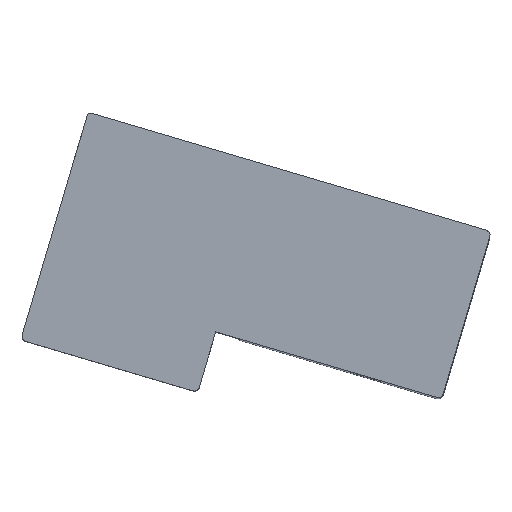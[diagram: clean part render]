
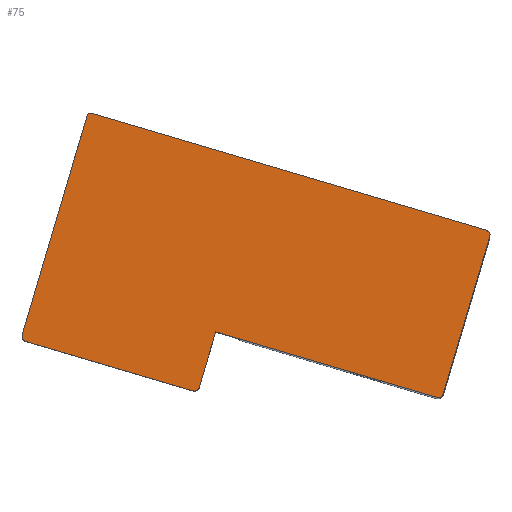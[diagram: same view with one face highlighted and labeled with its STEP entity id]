
A CAD part, top view. The second image highlights one B-rep face of the part: STEP entity #75.
In plain terms, the highlighted planar face has unit normal (0, 0, 1).
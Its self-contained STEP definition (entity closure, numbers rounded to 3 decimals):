
#22 = DIRECTION ( 'NONE',  ( 0., 0., -1. ) ) ;
#32 = EDGE_CURVE ( 'NONE', #1197, #1058, #312, .T. ) ;
#64 = ORIENTED_EDGE ( 'NONE', *, *, #1459, .F. ) ;
#72 = DIRECTION ( 'NONE',  ( -0.477, 0.879, 0. ) ) ;
#73 = DIRECTION ( 'NONE',  ( 0., 0., -1. ) ) ;
#75 = ADVANCED_FACE ( 'NONE', ( #539 ), #894, .F. ) ;
#135 = VECTOR ( 'NONE', #1700, 1000. ) ;
#195 = AXIS2_PLACEMENT_3D ( 'NONE', #910, #1368, #1363 ) ;
#199 = AXIS2_PLACEMENT_3D ( 'NONE', #1148, #73, #1041 ) ;
#220 = CIRCLE ( 'NONE', #1052, 0.15 ) ;
#256 = CARTESIAN_POINT ( 'NONE',  ( -35.314, -26.696, 19. ) ) ;
#312 = LINE ( 'NONE', #2003, #135 ) ;
#317 = EDGE_CURVE ( 'NONE', #1906, #722, #1544, .T. ) ;
#335 = VERTEX_POINT ( 'NONE', #377 ) ;
#338 = VERTEX_POINT ( 'NONE', #691 ) ;
#373 = VECTOR ( 'NONE', #1524, 1000. ) ;
#377 = CARTESIAN_POINT ( 'NONE',  ( -45.306, -26.891, 19. ) ) ;
#398 = VECTOR ( 'NONE', #870, 1000. ) ;
#465 = EDGE_CURVE ( 'NONE', #752, #1354, #775, .T. ) ;
#474 = CARTESIAN_POINT ( 'NONE',  ( -25.535, -29.332, 19. ) ) ;
#512 = AXIS2_PLACEMENT_3D ( 'NONE', #1888, #1242, #793 ) ;
#537 = ORIENTED_EDGE ( 'NONE', *, *, #1115, .F. ) ;
#539 = FACE_OUTER_BOUND ( 'NONE', #1815, .T. ) ;
#614 = CARTESIAN_POINT ( 'NONE',  ( -25.295, -29.403, 19. ) ) ;
#615 = ORIENTED_EDGE ( 'NONE', *, *, #727, .F. ) ;
#625 = LINE ( 'NONE', #635, #853 ) ;
#635 = CARTESIAN_POINT ( 'NONE',  ( -32.945, -18.688, 19. ) ) ;
#640 = DIRECTION ( 'NONE',  ( 0., 0., -1. ) ) ;
#643 = CARTESIAN_POINT ( 'NONE',  ( -25.606, -29.571, 19. ) ) ;
#646 = DIRECTION ( 'NONE',  ( 0.477, -0.879, 0. ) ) ;
#691 = CARTESIAN_POINT ( 'NONE',  ( -23.234, -21.565, 19. ) ) ;
#705 = CARTESIAN_POINT ( 'NONE',  ( -37.3, -29.262, 19. ) ) ;
#707 = VECTOR ( 'NONE', #1489, 1000. ) ;
#713 = CARTESIAN_POINT ( 'NONE',  ( -41.174, -12.062, 19. ) ) ;
#722 = VERTEX_POINT ( 'NONE', #1421 ) ;
#727 = EDGE_CURVE ( 'NONE', #335, #752, #2052, .T. ) ;
#733 = AXIS2_PLACEMENT_3D ( 'NONE', #474, #640, #646 ) ;
#746 = LINE ( 'NONE', #1653, #1629 ) ;
#752 = VERTEX_POINT ( 'NONE', #1112 ) ;
#775 = LINE ( 'NONE', #713, #398 ) ;
#793 = DIRECTION ( 'NONE',  ( -0.879, -0.477, 0. ) ) ;
#829 = CARTESIAN_POINT ( 'NONE',  ( -23.066, -21.875, 19. ) ) ;
#853 = VECTOR ( 'NONE', #960, 1000. ) ;
#870 = DIRECTION ( 'NONE',  ( 0.284, 0.959, 0. ) ) ;
#894 = PLANE ( 'NONE',  #195 ) ;
#910 = CARTESIAN_POINT ( 'NONE',  ( -34.82, -23.285, 19. ) ) ;
#960 = DIRECTION ( 'NONE',  ( 0.959, -0.284, 0. ) ) ;
#1041 = DIRECTION ( 'NONE',  ( 0.477, -0.879, 0. ) ) ;
#1052 = AXIS2_PLACEMENT_3D ( 'NONE', #1181, #2039, #72 ) ;
#1058 = VERTEX_POINT ( 'NONE', #614 ) ;
#1112 = CARTESIAN_POINT ( 'NONE',  ( -45.475, -26.58, 19. ) ) ;
#1115 = EDGE_CURVE ( 'NONE', #1252, #338, #625, .T. ) ;
#1148 = CARTESIAN_POINT ( 'NONE',  ( -37.229, -29.023, 19. ) ) ;
#1178 = EDGE_CURVE ( 'NONE', #338, #1197, #1529, .T. ) ;
#1181 = CARTESIAN_POINT ( 'NONE',  ( -42.214, -16.099, 19. ) ) ;
#1188 = CARTESIAN_POINT ( 'NONE',  ( -42.171, -15.955, 19. ) ) ;
#1197 = VERTEX_POINT ( 'NONE', #829 ) ;
#1242 = DIRECTION ( 'NONE',  ( 0., 0., -1. ) ) ;
#1252 = VERTEX_POINT ( 'NONE', #1188 ) ;
#1307 = ORIENTED_EDGE ( 'NONE', *, *, #2044, .F. ) ;
#1354 = VERTEX_POINT ( 'NONE', #1587 ) ;
#1356 = DIRECTION ( 'NONE',  ( -0.959, 0.284, 0. ) ) ;
#1363 = DIRECTION ( 'NONE',  ( 1., 0., 0. ) ) ;
#1368 = DIRECTION ( 'NONE',  ( 0., 0., -1. ) ) ;
#1371 = EDGE_CURVE ( 'NONE', #1058, #1981, #1682, .T. ) ;
#1394 = ORIENTED_EDGE ( 'NONE', *, *, #1371, .F. ) ;
#1421 = CARTESIAN_POINT ( 'NONE',  ( -36.989, -29.094, 19. ) ) ;
#1438 = CARTESIAN_POINT ( 'NONE',  ( -23.305, -21.804, 19. ) ) ;
#1454 = ORIENTED_EDGE ( 'NONE', *, *, #1719, .F. ) ;
#1459 = EDGE_CURVE ( 'NONE', #2068, #335, #746, .T. ) ;
#1484 = EDGE_CURVE ( 'NONE', #1981, #1906, #1786, .T. ) ;
#1489 = DIRECTION ( 'NONE',  ( -0.284, -0.959, 0. ) ) ;
#1524 = DIRECTION ( 'NONE',  ( -0.959, 0.284, 0. ) ) ;
#1529 = CIRCLE ( 'NONE', #2005, 0.25 ) ;
#1544 = LINE ( 'NONE', #1968, #707 ) ;
#1587 = CARTESIAN_POINT ( 'NONE',  ( -42.357, -16.056, 19. ) ) ;
#1590 = ORIENTED_EDGE ( 'NONE', *, *, #1178, .F. ) ;
#1629 = VECTOR ( 'NONE', #1356, 1000. ) ;
#1653 = CARTESIAN_POINT ( 'NONE',  ( -38.975, -28.766, 19. ) ) ;
#1682 = CIRCLE ( 'NONE', #733, 0.25 ) ;
#1700 = DIRECTION ( 'NONE',  ( -0.284, -0.959, 0. ) ) ;
#1719 = EDGE_CURVE ( 'NONE', #722, #2068, #1730, .T. ) ;
#1730 = CIRCLE ( 'NONE', #199, 0.25 ) ;
#1742 = ORIENTED_EDGE ( 'NONE', *, *, #1484, .F. ) ;
#1786 = LINE ( 'NONE', #256, #373 ) ;
#1804 = ORIENTED_EDGE ( 'NONE', *, *, #317, .F. ) ;
#1815 = EDGE_LOOP ( 'NONE', ( #615, #64, #1454, #1804, #1742, #1394, #2012, #1590, #537, #1307, #2034 ) ) ;
#1888 = CARTESIAN_POINT ( 'NONE',  ( -45.235, -26.651, 19. ) ) ;
#1890 = CARTESIAN_POINT ( 'NONE',  ( -36.201, -26.433, 19. ) ) ;
#1906 = VERTEX_POINT ( 'NONE', #1890 ) ;
#1923 = DIRECTION ( 'NONE',  ( 0.879, 0.477, 0. ) ) ;
#1968 = CARTESIAN_POINT ( 'NONE',  ( -34.849, -21.87, 19. ) ) ;
#1981 = VERTEX_POINT ( 'NONE', #643 ) ;
#2003 = CARTESIAN_POINT ( 'NONE',  ( -24.9, -28.067, 19. ) ) ;
#2005 = AXIS2_PLACEMENT_3D ( 'NONE', #1438, #22, #1923 ) ;
#2012 = ORIENTED_EDGE ( 'NONE', *, *, #32, .F. ) ;
#2034 = ORIENTED_EDGE ( 'NONE', *, *, #465, .F. ) ;
#2039 = DIRECTION ( 'NONE',  ( 0., 0., -1. ) ) ;
#2044 = EDGE_CURVE ( 'NONE', #1354, #1252, #220, .T. ) ;
#2052 = CIRCLE ( 'NONE', #512, 0.25 ) ;
#2068 = VERTEX_POINT ( 'NONE', #705 ) ;
